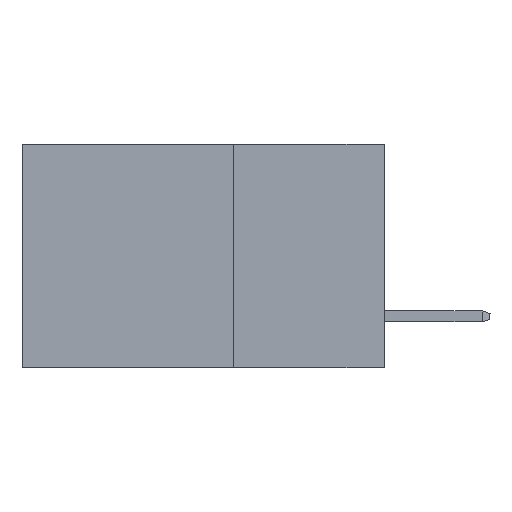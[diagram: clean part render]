
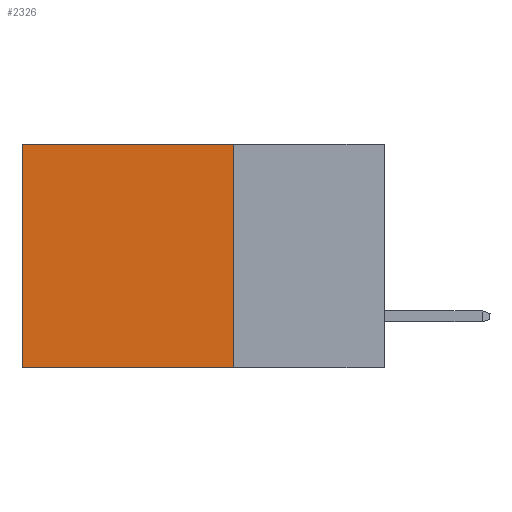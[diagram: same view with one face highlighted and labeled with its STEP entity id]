
A CAD part, left-side view. The second image highlights one B-rep face of the part: STEP entity #2326.
In plain terms, the highlighted planar face has unit normal (-1, 0, 0).
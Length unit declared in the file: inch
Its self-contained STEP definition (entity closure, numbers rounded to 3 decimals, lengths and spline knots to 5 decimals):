
#47 = VECTOR ( 'NONE', #3608, 39.37008 ) ;
#279 = ORIENTED_EDGE ( 'NONE', *, *, #1880, .F. ) ;
#681 = EDGE_CURVE ( 'NONE', #737, #1837, #5577, .T. ) ;
#737 = VERTEX_POINT ( 'NONE', #7167 ) ;
#850 = EDGE_LOOP ( 'NONE', ( #3325, #279, #3877, #2460 ) ) ;
#1033 = DIRECTION ( 'NONE',  ( 1., 0., 0. ) ) ;
#1693 = VERTEX_POINT ( 'NONE', #5477 ) ;
#1837 = VERTEX_POINT ( 'NONE', #5746 ) ;
#1880 = EDGE_CURVE ( 'NONE', #6029, #1693, #6992, .T. ) ;
#2326 = ADVANCED_FACE ( 'NONE', ( #5133 ), #3786, .F. ) ;
#2460 = ORIENTED_EDGE ( 'NONE', *, *, #681, .T. ) ;
#3020 = LINE ( 'NONE', #8326, #47 ) ;
#3325 = ORIENTED_EDGE ( 'NONE', *, *, #4430, .T. ) ;
#3608 = DIRECTION ( 'NONE',  ( 0., 0., -1. ) ) ;
#3693 = CARTESIAN_POINT ( 'NONE',  ( 0.2615, 0.25, -0.37 ) ) ;
#3786 = PLANE ( 'NONE',  #5221 ) ;
#3877 = ORIENTED_EDGE ( 'NONE', *, *, #4746, .F. ) ;
#3884 = DIRECTION ( 'NONE',  ( 0., 0., -1. ) ) ;
#4244 = DIRECTION ( 'NONE',  ( 0., 1., 0. ) ) ;
#4430 = EDGE_CURVE ( 'NONE', #1837, #1693, #3020, .T. ) ;
#4434 = CARTESIAN_POINT ( 'NONE',  ( 0.2615, 0.25, -0.37 ) ) ;
#4746 = EDGE_CURVE ( 'NONE', #737, #6029, #8551, .T. ) ;
#5133 = FACE_OUTER_BOUND ( 'NONE', #850, .T. ) ;
#5221 = AXIS2_PLACEMENT_3D ( 'NONE', #5891, #1033, #3884 ) ;
#5477 = CARTESIAN_POINT ( 'NONE',  ( 0.2615, 0.6, -0.37 ) ) ;
#5577 = LINE ( 'NONE', #8321, #6817 ) ;
#5746 = CARTESIAN_POINT ( 'NONE',  ( 0.2615, 0.6, 0. ) ) ;
#5891 = CARTESIAN_POINT ( 'NONE',  ( 0.2615, 0.25, -0.37 ) ) ;
#6029 = VERTEX_POINT ( 'NONE', #7942 ) ;
#6817 = VECTOR ( 'NONE', #4244, 39.37008 ) ;
#6992 = LINE ( 'NONE', #3693, #8133 ) ;
#7167 = CARTESIAN_POINT ( 'NONE',  ( 0.2615, 0.25, 0. ) ) ;
#7276 = DIRECTION ( 'NONE',  ( 0., 0., -1. ) ) ;
#7942 = CARTESIAN_POINT ( 'NONE',  ( 0.2615, 0.25, -0.37 ) ) ;
#8133 = VECTOR ( 'NONE', #8487, 39.37008 ) ;
#8321 = CARTESIAN_POINT ( 'NONE',  ( 0.2615, 0.25, 0. ) ) ;
#8326 = CARTESIAN_POINT ( 'NONE',  ( 0.2615, 0.6, -0.37 ) ) ;
#8487 = DIRECTION ( 'NONE',  ( 0., 1., 0. ) ) ;
#8551 = LINE ( 'NONE', #4434, #8814 ) ;
#8814 = VECTOR ( 'NONE', #7276, 39.37008 ) ;
